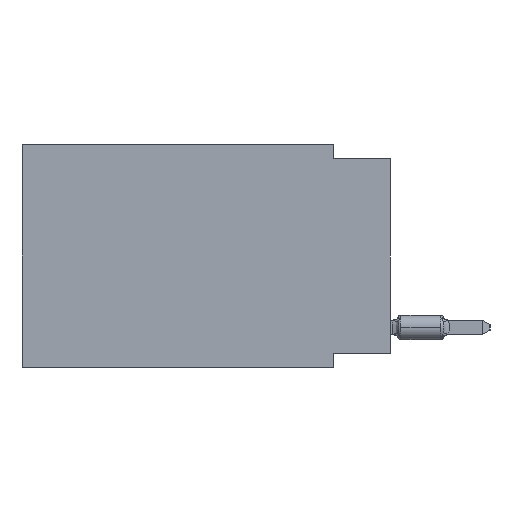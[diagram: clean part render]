
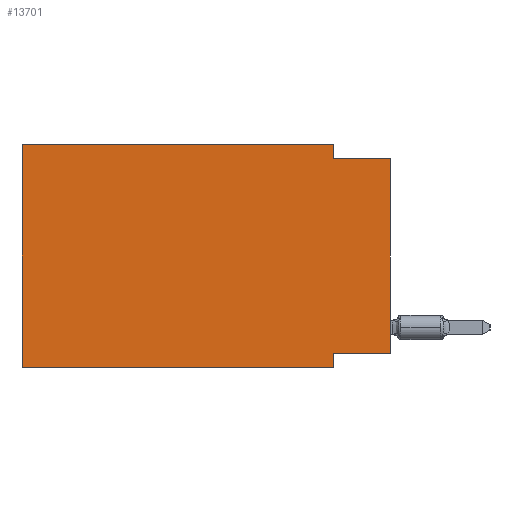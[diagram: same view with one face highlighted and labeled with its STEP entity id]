
A CAD part, left-side view. The second image highlights one B-rep face of the part: STEP entity #13701.
In plain terms, the highlighted planar face has unit normal (-1, 0, 0).
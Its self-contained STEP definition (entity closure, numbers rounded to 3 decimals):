
#133 = ORIENTED_EDGE ( 'NONE', *, *, #12269, .F. ) ;
#386 = EDGE_LOOP ( 'NONE', ( #20625, #15059, #17569, #5443, #17513, #1429, #8525, #133 ) ) ;
#467 = LINE ( 'NONE', #8217, #22953 ) ;
#1125 = CARTESIAN_POINT ( 'NONE',  ( 0., 2.54, -0.635 ) ) ;
#1137 = VERTEX_POINT ( 'NONE', #15665 ) ;
#1195 = EDGE_CURVE ( 'NONE', #1137, #19539, #5553, .T. ) ;
#1241 = AXIS2_PLACEMENT_3D ( 'NONE', #19244, #1860, #5782 ) ;
#1429 = ORIENTED_EDGE ( 'NONE', *, *, #1195, .T. ) ;
#1860 = DIRECTION ( 'NONE',  ( 1., 0., 0. ) ) ;
#3188 = LINE ( 'NONE', #24775, #7774 ) ;
#3457 = EDGE_CURVE ( 'NONE', #22803, #17494, #17233, .T. ) ;
#3774 = DIRECTION ( 'NONE',  ( 0., -1., 0. ) ) ;
#5443 = ORIENTED_EDGE ( 'NONE', *, *, #3457, .F. ) ;
#5553 = LINE ( 'NONE', #13289, #22975 ) ;
#5656 = PLANE ( 'NONE',  #1241 ) ;
#5782 = DIRECTION ( 'NONE',  ( 0., 0., -1. ) ) ;
#6059 = DIRECTION ( 'NONE',  ( 0., 0., -1. ) ) ;
#6304 = VECTOR ( 'NONE', #24598, 1000. ) ;
#7250 = DIRECTION ( 'NONE',  ( 0., 1., 0. ) ) ;
#7537 = CARTESIAN_POINT ( 'NONE',  ( 0., 0., -0.635 ) ) ;
#7774 = VECTOR ( 'NONE', #7250, 1000. ) ;
#8217 = CARTESIAN_POINT ( 'NONE',  ( 0., 2.54, -9.906 ) ) ;
#8400 = CARTESIAN_POINT ( 'NONE',  ( 0., 0., -0.635 ) ) ;
#8525 = ORIENTED_EDGE ( 'NONE', *, *, #8690, .F. ) ;
#8690 = EDGE_CURVE ( 'NONE', #15369, #19539, #467, .T. ) ;
#9481 = CARTESIAN_POINT ( 'NONE',  ( 0., 0., 0. ) ) ;
#9982 = CARTESIAN_POINT ( 'NONE',  ( 0., 16.383, 0. ) ) ;
#11511 = DIRECTION ( 'NONE',  ( 0., 0., 1. ) ) ;
#12269 = EDGE_CURVE ( 'NONE', #22971, #15369, #3188, .T. ) ;
#12911 = LINE ( 'NONE', #9481, #6304 ) ;
#12998 = DIRECTION ( 'NONE',  ( 0., 0., -1. ) ) ;
#13289 = CARTESIAN_POINT ( 'NONE',  ( 0., 16.383, -9.906 ) ) ;
#13651 = LINE ( 'NONE', #9982, #22752 ) ;
#13701 = ADVANCED_FACE ( 'NONE', ( #23184 ), #5656, .F. ) ;
#13756 = VECTOR ( 'NONE', #12998, 1000. ) ;
#14055 = EDGE_CURVE ( 'NONE', #21399, #22526, #19102, .T. ) ;
#14181 = CARTESIAN_POINT ( 'NONE',  ( 0., 2.54, 0. ) ) ;
#14319 = VECTOR ( 'NONE', #3774, 1000. ) ;
#15059 = ORIENTED_EDGE ( 'NONE', *, *, #14055, .F. ) ;
#15150 = EDGE_CURVE ( 'NONE', #17494, #21399, #16096, .T. ) ;
#15153 = DIRECTION ( 'NONE',  ( 0., -1., 0. ) ) ;
#15369 = VERTEX_POINT ( 'NONE', #23527 ) ;
#15665 = CARTESIAN_POINT ( 'NONE',  ( 0., 16.383, -9.906 ) ) ;
#16069 = CARTESIAN_POINT ( 'NONE',  ( 0., 2.54, -9.906 ) ) ;
#16096 = LINE ( 'NONE', #14181, #13756 ) ;
#17233 = LINE ( 'NONE', #24989, #14319 ) ;
#17305 = CARTESIAN_POINT ( 'NONE',  ( 0., 2.54, 0. ) ) ;
#17494 = VERTEX_POINT ( 'NONE', #17305 ) ;
#17513 = ORIENTED_EDGE ( 'NONE', *, *, #20539, .F. ) ;
#17569 = ORIENTED_EDGE ( 'NONE', *, *, #15150, .F. ) ;
#19102 = LINE ( 'NONE', #7537, #23950 ) ;
#19244 = CARTESIAN_POINT ( 'NONE',  ( 0., 16.383, 0. ) ) ;
#19539 = VERTEX_POINT ( 'NONE', #16069 ) ;
#20539 = EDGE_CURVE ( 'NONE', #1137, #22803, #13651, .T. ) ;
#20625 = ORIENTED_EDGE ( 'NONE', *, *, #24173, .T. ) ;
#21035 = DIRECTION ( 'NONE',  ( 0., -1., 0. ) ) ;
#21399 = VERTEX_POINT ( 'NONE', #1125 ) ;
#22526 = VERTEX_POINT ( 'NONE', #8400 ) ;
#22610 = CARTESIAN_POINT ( 'NONE',  ( 0., 16.383, 0. ) ) ;
#22752 = VECTOR ( 'NONE', #11511, 1000. ) ;
#22803 = VERTEX_POINT ( 'NONE', #22610 ) ;
#22953 = VECTOR ( 'NONE', #6059, 1000. ) ;
#22971 = VERTEX_POINT ( 'NONE', #23357 ) ;
#22975 = VECTOR ( 'NONE', #21035, 1000. ) ;
#23184 = FACE_OUTER_BOUND ( 'NONE', #386, .T. ) ;
#23357 = CARTESIAN_POINT ( 'NONE',  ( 0., 0., -9.271 ) ) ;
#23527 = CARTESIAN_POINT ( 'NONE',  ( 0., 2.54, -9.271 ) ) ;
#23950 = VECTOR ( 'NONE', #15153, 1000. ) ;
#24173 = EDGE_CURVE ( 'NONE', #22971, #22526, #12911, .T. ) ;
#24598 = DIRECTION ( 'NONE',  ( 0., 0., 1. ) ) ;
#24775 = CARTESIAN_POINT ( 'NONE',  ( 0., 0., -9.271 ) ) ;
#24989 = CARTESIAN_POINT ( 'NONE',  ( 0., 16.383, 0. ) ) ;
